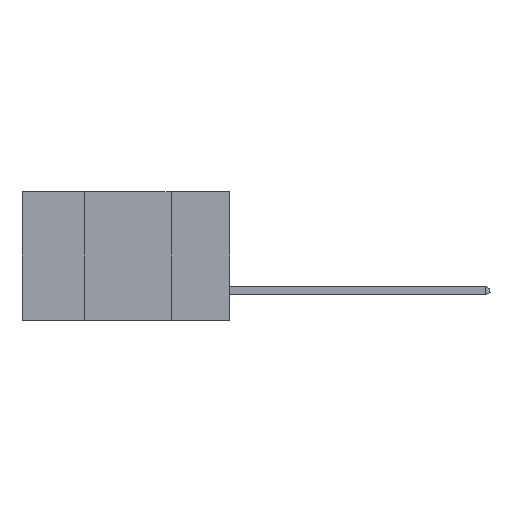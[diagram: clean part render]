
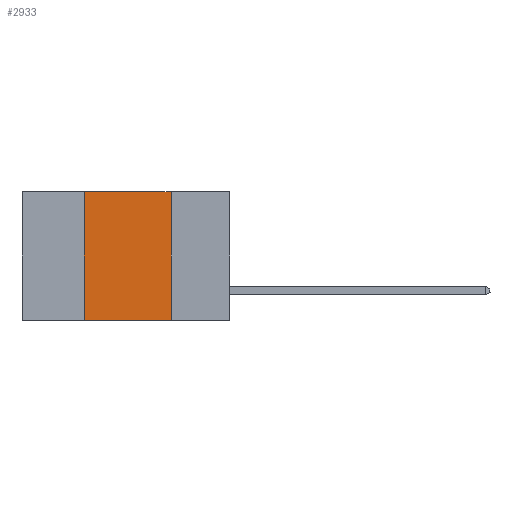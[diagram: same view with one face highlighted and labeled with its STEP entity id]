
A CAD part, left-side view. The second image highlights one B-rep face of the part: STEP entity #2933.
In plain terms, the highlighted planar face has unit normal (-1, 0, 0).
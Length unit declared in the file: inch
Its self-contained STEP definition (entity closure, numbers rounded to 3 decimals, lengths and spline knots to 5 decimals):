
#385 = CARTESIAN_POINT ( 'NONE',  ( 0., 0.17, 0. ) ) ;
#430 = DIRECTION ( 'NONE',  ( 0., -1., 0. ) ) ;
#484 = CARTESIAN_POINT ( 'NONE',  ( 0., 0.42, 0. ) ) ;
#768 = ORIENTED_EDGE ( 'NONE', *, *, #7756, .T. ) ;
#971 = DIRECTION ( 'NONE',  ( 0., 0., -1. ) ) ;
#1225 = ORIENTED_EDGE ( 'NONE', *, *, #12614, .F. ) ;
#1736 = DIRECTION ( 'NONE',  ( 0., 0., 1. ) ) ;
#2019 = VECTOR ( 'NONE', #1736, 39.37008 ) ;
#2470 = LINE ( 'NONE', #2481, #7321 ) ;
#2481 = CARTESIAN_POINT ( 'NONE',  ( 0., 0.17, 0. ) ) ;
#2496 = VERTEX_POINT ( 'NONE', #14643 ) ;
#2653 = ORIENTED_EDGE ( 'NONE', *, *, #4437, .F. ) ;
#2738 = VERTEX_POINT ( 'NONE', #385 ) ;
#2742 = EDGE_CURVE ( 'NONE', #6547, #2496, #6163, .T. ) ;
#2933 = ADVANCED_FACE ( 'NONE', ( #7222 ), #5593, .F. ) ;
#3768 = AXIS2_PLACEMENT_3D ( 'NONE', #13520, #6708, #971 ) ;
#4035 = CARTESIAN_POINT ( 'NONE',  ( 0., 0.17, -0.37 ) ) ;
#4437 = EDGE_CURVE ( 'NONE', #2496, #2738, #12678, .T. ) ;
#4926 = DIRECTION ( 'NONE',  ( 0., -1., 0. ) ) ;
#5224 = LINE ( 'NONE', #10619, #8786 ) ;
#5593 = PLANE ( 'NONE',  #3768 ) ;
#6161 = CARTESIAN_POINT ( 'NONE',  ( 0., 0.6, 0. ) ) ;
#6163 = LINE ( 'NONE', #484, #2019 ) ;
#6547 = VERTEX_POINT ( 'NONE', #13012 ) ;
#6708 = DIRECTION ( 'NONE',  ( 1., 0., 0. ) ) ;
#7222 = FACE_OUTER_BOUND ( 'NONE', #12507, .T. ) ;
#7321 = VECTOR ( 'NONE', #12636, 39.37008 ) ;
#7756 = EDGE_CURVE ( 'NONE', #6547, #7849, #5224, .T. ) ;
#7849 = VERTEX_POINT ( 'NONE', #4035 ) ;
#8229 = VECTOR ( 'NONE', #430, 39.37008 ) ;
#8786 = VECTOR ( 'NONE', #4926, 39.37008 ) ;
#10619 = CARTESIAN_POINT ( 'NONE',  ( 0., 0.6, -0.37 ) ) ;
#11104 = ORIENTED_EDGE ( 'NONE', *, *, #2742, .F. ) ;
#12507 = EDGE_LOOP ( 'NONE', ( #1225, #2653, #11104, #768 ) ) ;
#12614 = EDGE_CURVE ( 'NONE', #2738, #7849, #2470, .T. ) ;
#12636 = DIRECTION ( 'NONE',  ( 0., 0., -1. ) ) ;
#12678 = LINE ( 'NONE', #6161, #8229 ) ;
#13012 = CARTESIAN_POINT ( 'NONE',  ( 0., 0.42, -0.37 ) ) ;
#13520 = CARTESIAN_POINT ( 'NONE',  ( 0., 0.6, 0. ) ) ;
#14643 = CARTESIAN_POINT ( 'NONE',  ( 0., 0.42, 0. ) ) ;
